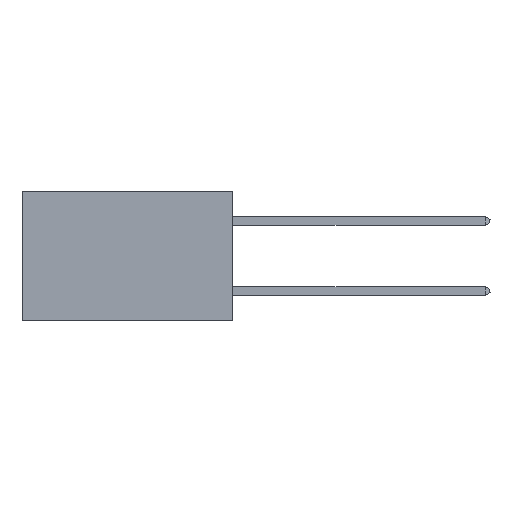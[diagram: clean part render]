
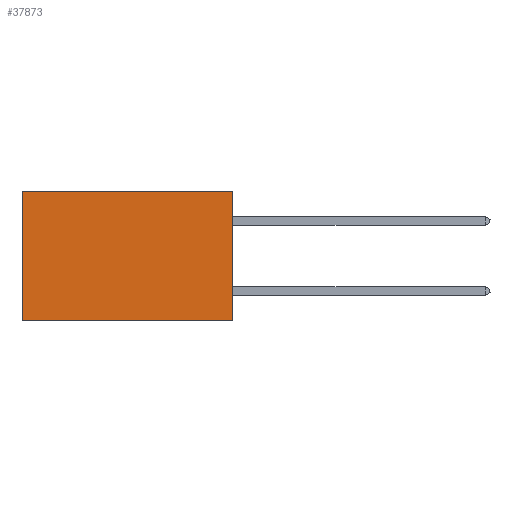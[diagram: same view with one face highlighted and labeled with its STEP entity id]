
A CAD part, left-side view. The second image highlights one B-rep face of the part: STEP entity #37873.
In plain terms, the highlighted planar face has unit normal (-1, 0, 0).
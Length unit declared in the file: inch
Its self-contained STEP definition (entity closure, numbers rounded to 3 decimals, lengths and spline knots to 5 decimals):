
#557 = LINE ( 'NONE', #13275, #21462 ) ;
#1059 = CARTESIAN_POINT ( 'NONE',  ( 0.2875, 0., 0. ) ) ;
#2472 = EDGE_CURVE ( 'NONE', #27647, #24172, #16178, .T. ) ;
#2884 = CARTESIAN_POINT ( 'NONE',  ( 0.2875, 0., -0.37 ) ) ;
#3901 = CARTESIAN_POINT ( 'NONE',  ( 0.2875, 0.6, -0.37 ) ) ;
#5268 = LINE ( 'NONE', #1059, #13991 ) ;
#6656 = CARTESIAN_POINT ( 'NONE',  ( 0.2875, 0., 0. ) ) ;
#6916 = ORIENTED_EDGE ( 'NONE', *, *, #2472, .F. ) ;
#7892 = CARTESIAN_POINT ( 'NONE',  ( 0.2875, 0.6, 0. ) ) ;
#8717 = DIRECTION ( 'NONE',  ( 0., 1., 0. ) ) ;
#11115 = CARTESIAN_POINT ( 'NONE',  ( 0.2875, 0., 0. ) ) ;
#11215 = ORIENTED_EDGE ( 'NONE', *, *, #25798, .F. ) ;
#11532 = FACE_OUTER_BOUND ( 'NONE', #42611, .T. ) ;
#13275 = CARTESIAN_POINT ( 'NONE',  ( 0.2875, 0., 0. ) ) ;
#13593 = ORIENTED_EDGE ( 'NONE', *, *, #18053, .T. ) ;
#13942 = ORIENTED_EDGE ( 'NONE', *, *, #25107, .T. ) ;
#13991 = VECTOR ( 'NONE', #8717, 39.37008 ) ;
#14854 = LINE ( 'NONE', #34599, #39211 ) ;
#16178 = LINE ( 'NONE', #2884, #23715 ) ;
#17276 = CARTESIAN_POINT ( 'NONE',  ( 0.2875, 0., -0.37 ) ) ;
#18053 = EDGE_CURVE ( 'NONE', #20229, #24172, #14854, .T. ) ;
#18531 = DIRECTION ( 'NONE',  ( 0., 0., -1. ) ) ;
#20215 = DIRECTION ( 'NONE',  ( 0., 0., -1. ) ) ;
#20229 = VERTEX_POINT ( 'NONE', #7892 ) ;
#21462 = VECTOR ( 'NONE', #20215, 39.37008 ) ;
#23715 = VECTOR ( 'NONE', #36824, 39.37008 ) ;
#24172 = VERTEX_POINT ( 'NONE', #3901 ) ;
#25107 = EDGE_CURVE ( 'NONE', #38902, #20229, #5268, .T. ) ;
#25798 = EDGE_CURVE ( 'NONE', #38902, #27647, #557, .T. ) ;
#27647 = VERTEX_POINT ( 'NONE', #17276 ) ;
#30222 = DIRECTION ( 'NONE',  ( 1., 0., 0. ) ) ;
#34599 = CARTESIAN_POINT ( 'NONE',  ( 0.2875, 0.6, 0. ) ) ;
#36824 = DIRECTION ( 'NONE',  ( 0., 1., 0. ) ) ;
#37873 = ADVANCED_FACE ( 'NONE', ( #11532 ), #41083, .F. ) ;
#38902 = VERTEX_POINT ( 'NONE', #6656 ) ;
#39211 = VECTOR ( 'NONE', #42044, 39.37008 ) ;
#40978 = AXIS2_PLACEMENT_3D ( 'NONE', #11115, #30222, #18531 ) ;
#41083 = PLANE ( 'NONE',  #40978 ) ;
#42044 = DIRECTION ( 'NONE',  ( 0., 0., -1. ) ) ;
#42611 = EDGE_LOOP ( 'NONE', ( #13593, #6916, #11215, #13942 ) ) ;
